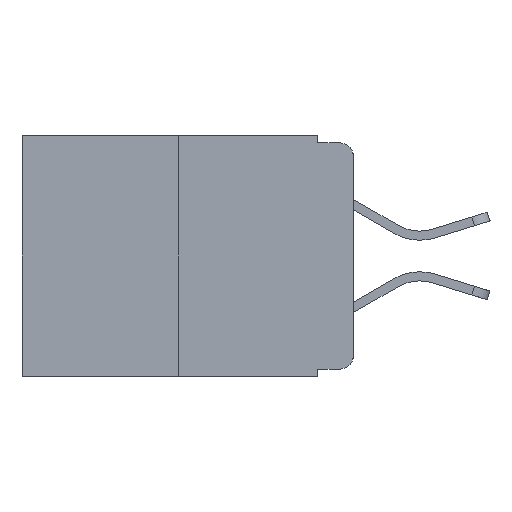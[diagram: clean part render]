
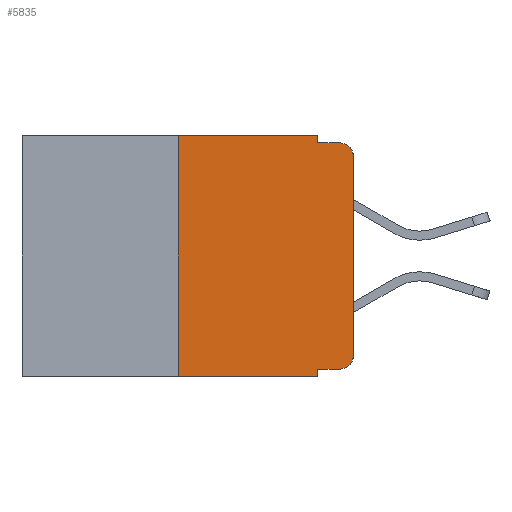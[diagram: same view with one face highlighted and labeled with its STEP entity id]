
A CAD part, left-side view. The second image highlights one B-rep face of the part: STEP entity #5835.
In plain terms, the highlighted planar face has unit normal (-1, 0, 0).
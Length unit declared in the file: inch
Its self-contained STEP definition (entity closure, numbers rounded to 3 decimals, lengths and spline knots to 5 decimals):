
#183 = CARTESIAN_POINT ( 'NONE',  ( 0., 0.051, 0. ) ) ;
#319 = ORIENTED_EDGE ( 'NONE', *, *, #5775, .F. ) ;
#535 = ORIENTED_EDGE ( 'NONE', *, *, #9631, .T. ) ;
#594 = CARTESIAN_POINT ( 'NONE',  ( 0., 0.051, -0.01 ) ) ;
#927 = DIRECTION ( 'NONE',  ( 0., -1., 0. ) ) ;
#940 = VERTEX_POINT ( 'NONE', #594 ) ;
#1081 = ORIENTED_EDGE ( 'NONE', *, *, #2259, .F. ) ;
#1097 = CARTESIAN_POINT ( 'NONE',  ( 0., 0.02, -0.03 ) ) ;
#1250 = VECTOR ( 'NONE', #8333, 39.37008 ) ;
#1373 = ORIENTED_EDGE ( 'NONE', *, *, #3175, .T. ) ;
#1376 = CARTESIAN_POINT ( 'NONE',  ( 0., 0., 0. ) ) ;
#1428 = DIRECTION ( 'NONE',  ( 0., 0., 1. ) ) ;
#1523 = VERTEX_POINT ( 'NONE', #10120 ) ;
#1556 = ORIENTED_EDGE ( 'NONE', *, *, #1715, .F. ) ;
#1591 = DIRECTION ( 'NONE',  ( 0., -1., 0. ) ) ;
#1664 = DIRECTION ( 'NONE',  ( 0., 0., -1. ) ) ;
#1710 = EDGE_CURVE ( 'NONE', #940, #1523, #6898, .T. ) ;
#1715 = EDGE_CURVE ( 'NONE', #8474, #3459, #11263, .T. ) ;
#1916 = CARTESIAN_POINT ( 'NONE',  ( 0., 0.473, 0. ) ) ;
#2070 = CARTESIAN_POINT ( 'NONE',  ( 0., 0.473, -0.343 ) ) ;
#2259 = EDGE_CURVE ( 'NONE', #8710, #940, #11123, .T. ) ;
#2407 = ORIENTED_EDGE ( 'NONE', *, *, #11252, .T. ) ;
#2473 = CARTESIAN_POINT ( 'NONE',  ( 0., 0.02, -0.333 ) ) ;
#2655 = CARTESIAN_POINT ( 'NONE',  ( 0., 0.051, -0.333 ) ) ;
#3106 = VECTOR ( 'NONE', #3760, 39.37008 ) ;
#3175 = EDGE_CURVE ( 'NONE', #4131, #3408, #5235, .T. ) ;
#3408 = VERTEX_POINT ( 'NONE', #6488 ) ;
#3457 = CARTESIAN_POINT ( 'NONE',  ( 0., 0.051, -0.01 ) ) ;
#3459 = VERTEX_POINT ( 'NONE', #6177 ) ;
#3645 = CARTESIAN_POINT ( 'NONE',  ( 0., 0.051, 0. ) ) ;
#3760 = DIRECTION ( 'NONE',  ( 0., 0., -1. ) ) ;
#3937 = DIRECTION ( 'NONE',  ( -1., 0., 0. ) ) ;
#4131 = VERTEX_POINT ( 'NONE', #2473 ) ;
#4345 = ORIENTED_EDGE ( 'NONE', *, *, #5178, .T. ) ;
#4428 = CARTESIAN_POINT ( 'NONE',  ( 0., 0.25, 0. ) ) ;
#4699 = VECTOR ( 'NONE', #9425, 39.37008 ) ;
#4758 = VECTOR ( 'NONE', #9573, 39.37008 ) ;
#4780 = DIRECTION ( 'NONE',  ( 1., 0., 0. ) ) ;
#4889 = FACE_OUTER_BOUND ( 'NONE', #6181, .T. ) ;
#5178 = EDGE_CURVE ( 'NONE', #10967, #4131, #9447, .T. ) ;
#5235 = CIRCLE ( 'NONE', #8873, 0.02 ) ;
#5373 = LINE ( 'NONE', #1916, #11177 ) ;
#5436 = VECTOR ( 'NONE', #1428, 39.37008 ) ;
#5465 = LINE ( 'NONE', #183, #3106 ) ;
#5641 = DIRECTION ( 'NONE',  ( 0., 0., -1. ) ) ;
#5647 = ORIENTED_EDGE ( 'NONE', *, *, #6273, .T. ) ;
#5690 = CARTESIAN_POINT ( 'NONE',  ( 0., 0.473, 0. ) ) ;
#5753 = LINE ( 'NONE', #1376, #5436 ) ;
#5775 = EDGE_CURVE ( 'NONE', #10967, #8062, #5465, .T. ) ;
#5835 = ADVANCED_FACE ( 'NONE', ( #4889 ), #7431, .F. ) ;
#5923 = DIRECTION ( 'NONE',  ( -1., 0., 0. ) ) ;
#6177 = CARTESIAN_POINT ( 'NONE',  ( 0., 0.25, 0. ) ) ;
#6181 = EDGE_LOOP ( 'NONE', ( #535, #2407, #9452, #1081, #6362, #1556, #5647, #319, #4345, #1373 ) ) ;
#6273 = EDGE_CURVE ( 'NONE', #8474, #8062, #9230, .T. ) ;
#6362 = ORIENTED_EDGE ( 'NONE', *, *, #7029, .F. ) ;
#6488 = CARTESIAN_POINT ( 'NONE',  ( 0., 0., -0.313 ) ) ;
#6556 = DIRECTION ( 'NONE',  ( 0., 0., -1. ) ) ;
#6862 = CARTESIAN_POINT ( 'NONE',  ( 0., 0.051, -0.333 ) ) ;
#6898 = LINE ( 'NONE', #3457, #8238 ) ;
#6912 = CARTESIAN_POINT ( 'NONE',  ( 0., 0.02, -0.313 ) ) ;
#6994 = CARTESIAN_POINT ( 'NONE',  ( 0., 0., -0.03 ) ) ;
#7029 = EDGE_CURVE ( 'NONE', #3459, #8710, #5373, .T. ) ;
#7067 = DIRECTION ( 'NONE',  ( 0., -1., 0. ) ) ;
#7111 = VERTEX_POINT ( 'NONE', #6994 ) ;
#7322 = AXIS2_PLACEMENT_3D ( 'NONE', #5690, #4780, #6556 ) ;
#7392 = CARTESIAN_POINT ( 'NONE',  ( 0., 0.25, -0.343 ) ) ;
#7431 = PLANE ( 'NONE',  #7322 ) ;
#8062 = VERTEX_POINT ( 'NONE', #9963 ) ;
#8115 = AXIS2_PLACEMENT_3D ( 'NONE', #1097, #3937, #5641 ) ;
#8238 = VECTOR ( 'NONE', #1591, 39.37008 ) ;
#8297 = CIRCLE ( 'NONE', #8115, 0.02 ) ;
#8333 = DIRECTION ( 'NONE',  ( 0., -1., 0. ) ) ;
#8474 = VERTEX_POINT ( 'NONE', #7392 ) ;
#8710 = VERTEX_POINT ( 'NONE', #3645 ) ;
#8873 = AXIS2_PLACEMENT_3D ( 'NONE', #6912, #5923, #1664 ) ;
#9230 = LINE ( 'NONE', #2070, #1250 ) ;
#9425 = DIRECTION ( 'NONE',  ( 0., 0., -1. ) ) ;
#9447 = LINE ( 'NONE', #2655, #10790 ) ;
#9452 = ORIENTED_EDGE ( 'NONE', *, *, #1710, .F. ) ;
#9477 = CARTESIAN_POINT ( 'NONE',  ( 0., 0.051, 0. ) ) ;
#9573 = DIRECTION ( 'NONE',  ( 0., 0., 1. ) ) ;
#9631 = EDGE_CURVE ( 'NONE', #3408, #7111, #5753, .T. ) ;
#9963 = CARTESIAN_POINT ( 'NONE',  ( 0., 0.051, -0.343 ) ) ;
#10120 = CARTESIAN_POINT ( 'NONE',  ( 0., 0.02, -0.01 ) ) ;
#10790 = VECTOR ( 'NONE', #7067, 39.37008 ) ;
#10967 = VERTEX_POINT ( 'NONE', #6862 ) ;
#11123 = LINE ( 'NONE', #9477, #4699 ) ;
#11177 = VECTOR ( 'NONE', #927, 39.37008 ) ;
#11252 = EDGE_CURVE ( 'NONE', #7111, #1523, #8297, .T. ) ;
#11263 = LINE ( 'NONE', #4428, #4758 ) ;
